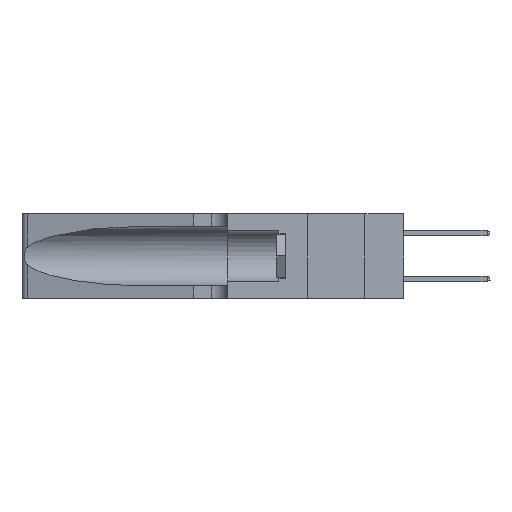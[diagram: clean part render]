
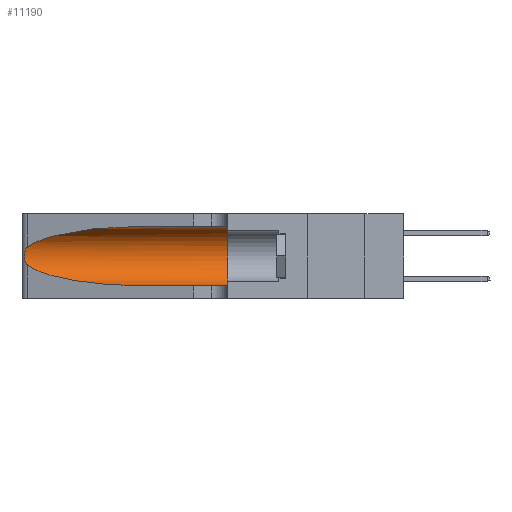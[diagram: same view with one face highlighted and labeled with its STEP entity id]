
A CAD part, left-side view. The second image highlights one B-rep face of the part: STEP entity #11190.
In plain terms, the highlighted cylindrical face has radius 3.308 mm (diameter 6.617 mm), a partial arc.
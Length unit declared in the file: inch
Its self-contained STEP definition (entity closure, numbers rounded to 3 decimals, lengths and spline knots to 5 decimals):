
#15 = VECTOR ( 'NONE', #9823, 39.37008 ) ;
#392 = CARTESIAN_POINT ( 'NONE',  ( 0.25487, 1.22718, 0.14631 ) ) ;
#476 = CARTESIAN_POINT ( 'NONE',  ( 0.25487, 1.22718, 0.22369 ) ) ;
#621 = CARTESIAN_POINT ( 'NONE',  ( 0.26075, 1.23896, 0.19203 ) ) ;
#923 = B_SPLINE_CURVE_WITH_KNOTS ( 'NONE', 3,
 ( #476, #33940, #37193, #17357, #40486, #20738, #621, #24098, #4018, #27424, #7390, #30756, #10779, #34089 ),
 .UNSPECIFIED., .F., .F.,
 ( 4, 2, 2, 2, 2, 2, 4 ),
 ( 0., 0.00027, 0.00053, 0.00107, 0.0016, 0.00187, 0.00214 ),
 .UNSPECIFIED. ) ;
#2087 = CARTESIAN_POINT ( 'NONE',  ( 0.2373, 1.15595, 0.28018 ) ) ;
#2891 = EDGE_CURVE ( 'NONE', #39879, #36995, #35555, .T. ) ;
#3802 = CARTESIAN_POINT ( 'NONE',  ( 0.18966, 0.96281, 0.05475 ) ) ;
#4015 = VERTEX_POINT ( 'NONE', #32799 ) ;
#4018 = CARTESIAN_POINT ( 'NONE',  ( 0.26017, 1.23833, 0.17102 ) ) ;
#5303 = DIRECTION ( 'NONE',  ( 0., 0., -1. ) ) ;
#5999 = CARTESIAN_POINT ( 'NONE',  ( 0.25487, 1.22718, 0.14631 ) ) ;
#7390 = CARTESIAN_POINT ( 'NONE',  ( 0.25789, 1.23486, 0.15765 ) ) ;
#7805 = CYLINDRICAL_SURFACE ( 'NONE', #13889, 0.13025 ) ;
#8753 =( BOUNDED_CURVE ( )  B_SPLINE_CURVE ( 3, ( #18828, #38622, #2087, #25556 ),
 .UNSPECIFIED., .F., .T. ) 
 B_SPLINE_CURVE_WITH_KNOTS ( ( 4, 4 ),
 ( 1.5708, 2.84003 ),
 .UNSPECIFIED. ) 
 CURVE ( )  GEOMETRIC_REPRESENTATION_ITEM ( )  RATIONAL_B_SPLINE_CURVE ( ( 1., 0.87, 0.87, 1. ) ) 
 REPRESENTATION_ITEM ( '' )  );
#9823 = DIRECTION ( 'NONE',  ( 0., -1., 0. ) ) ;
#10285 = ORIENTED_EDGE ( 'NONE', *, *, #17735, .T. ) ;
#10708 = LINE ( 'NONE', #40584, #28474 ) ;
#10779 = CARTESIAN_POINT ( 'NONE',  ( 0.25555, 1.22993, 0.14849 ) ) ;
#11106 = CARTESIAN_POINT ( 'NONE',  ( 0.25487, 1.22718, 0.22369 ) ) ;
#11190 = ADVANCED_FACE ( 'NONE', ( #17780 ), #7805, .F. ) ;
#11629 = VERTEX_POINT ( 'NONE', #5999 ) ;
#12358 = AXIS2_PLACEMENT_3D ( 'NONE', #17512, #40625, #20872 ) ;
#13596 = CARTESIAN_POINT ( 'NONE',  ( 0.1305, 0.35, 0.05475 ) ) ;
#13766 = ORIENTED_EDGE ( 'NONE', *, *, #23562, .T. ) ;
#13889 = AXIS2_PLACEMENT_3D ( 'NONE', #15247, #25363, #5303 ) ;
#15247 = CARTESIAN_POINT ( 'NONE',  ( 0.1305, 1.61858, 0.185 ) ) ;
#16283 = CARTESIAN_POINT ( 'NONE',  ( 0.1305, 0.35, 0.31525 ) ) ;
#16399 = ORIENTED_EDGE ( 'NONE', *, *, #24608, .T. ) ;
#16413 = VERTEX_POINT ( 'NONE', #11106 ) ;
#17134 = CARTESIAN_POINT ( 'NONE',  ( 0.2373, 1.15595, 0.08982 ) ) ;
#17357 = CARTESIAN_POINT ( 'NONE',  ( 0.25787, 1.23484, 0.2124 ) ) ;
#17512 = CARTESIAN_POINT ( 'NONE',  ( 0.1305, 0.35, 0.185 ) ) ;
#17735 = EDGE_CURVE ( 'NONE', #11629, #39879, #39597, .T. ) ;
#17780 = FACE_OUTER_BOUND ( 'NONE', #39737, .T. ) ;
#18193 = ORIENTED_EDGE ( 'NONE', *, *, #39447, .F. ) ;
#18828 = CARTESIAN_POINT ( 'NONE',  ( 0.1305, 0.72297, 0.31525 ) ) ;
#20738 = CARTESIAN_POINT ( 'NONE',  ( 0.26018, 1.23835, 0.19895 ) ) ;
#20794 = ORIENTED_EDGE ( 'NONE', *, *, #2891, .T. ) ;
#20834 = DIRECTION ( 'NONE',  ( 0., -1., 0. ) ) ;
#20872 = DIRECTION ( 'NONE',  ( 0., 0., 1. ) ) ;
#23562 = EDGE_CURVE ( 'NONE', #4015, #16413, #8753, .T. ) ;
#24098 = CARTESIAN_POINT ( 'NONE',  ( 0.26075, 1.23896, 0.178 ) ) ;
#24608 = EDGE_CURVE ( 'NONE', #16413, #11629, #923, .T. ) ;
#25363 = DIRECTION ( 'NONE',  ( 0., -1., 0. ) ) ;
#25556 = CARTESIAN_POINT ( 'NONE',  ( 0.25487, 1.22718, 0.22369 ) ) ;
#25918 = CIRCLE ( 'NONE', #12358, 0.13025 ) ;
#26651 = CARTESIAN_POINT ( 'NONE',  ( 0.1305, 1.61858, 0.05475 ) ) ;
#27219 = CARTESIAN_POINT ( 'NONE',  ( 0.1305, 0.72297, 0.05475 ) ) ;
#27424 = CARTESIAN_POINT ( 'NONE',  ( 0.25856, 1.23593, 0.16098 ) ) ;
#28474 = VECTOR ( 'NONE', #20834, 39.37008 ) ;
#30756 = CARTESIAN_POINT ( 'NONE',  ( 0.25639, 1.23186, 0.15144 ) ) ;
#32799 = CARTESIAN_POINT ( 'NONE',  ( 0.1305, 0.72297, 0.31525 ) ) ;
#33940 = CARTESIAN_POINT ( 'NONE',  ( 0.25555, 1.22994, 0.2215 ) ) ;
#34089 = CARTESIAN_POINT ( 'NONE',  ( 0.25487, 1.22718, 0.14631 ) ) ;
#35555 = LINE ( 'NONE', #26651, #15 ) ;
#36995 = VERTEX_POINT ( 'NONE', #13596 ) ;
#37193 = CARTESIAN_POINT ( 'NONE',  ( 0.25639, 1.23184, 0.21858 ) ) ;
#38063 = VERTEX_POINT ( 'NONE', #16283 ) ;
#38622 = CARTESIAN_POINT ( 'NONE',  ( 0.18966, 0.96281, 0.31525 ) ) ;
#39397 = CARTESIAN_POINT ( 'NONE',  ( 0.1305, 0.72297, 0.05475 ) ) ;
#39447 = EDGE_CURVE ( 'NONE', #4015, #38063, #10708, .T. ) ;
#39597 =( BOUNDED_CURVE ( )  B_SPLINE_CURVE ( 3, ( #392, #17134, #3802, #27219 ),
 .UNSPECIFIED., .F., .T. ) 
 B_SPLINE_CURVE_WITH_KNOTS ( ( 4, 4 ),
 ( 3.44316, 4.71239 ),
 .UNSPECIFIED. ) 
 CURVE ( )  GEOMETRIC_REPRESENTATION_ITEM ( )  RATIONAL_B_SPLINE_CURVE ( ( 1., 0.87, 0.87, 1. ) ) 
 REPRESENTATION_ITEM ( '' )  );
#39737 = EDGE_LOOP ( 'NONE', ( #13766, #16399, #10285, #20794, #41947, #18193 ) ) ;
#39879 = VERTEX_POINT ( 'NONE', #39397 ) ;
#40486 = CARTESIAN_POINT ( 'NONE',  ( 0.25854, 1.2359, 0.20912 ) ) ;
#40584 = CARTESIAN_POINT ( 'NONE',  ( 0.1305, 1.61858, 0.31525 ) ) ;
#40625 = DIRECTION ( 'NONE',  ( 0., 1., 0. ) ) ;
#40741 = EDGE_CURVE ( 'NONE', #38063, #36995, #25918, .T. ) ;
#41947 = ORIENTED_EDGE ( 'NONE', *, *, #40741, .F. ) ;
